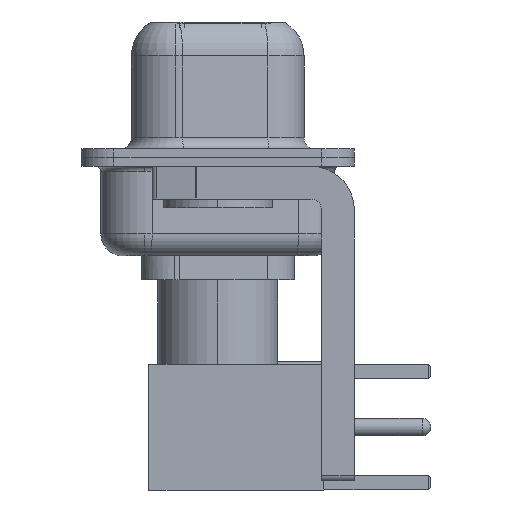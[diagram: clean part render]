
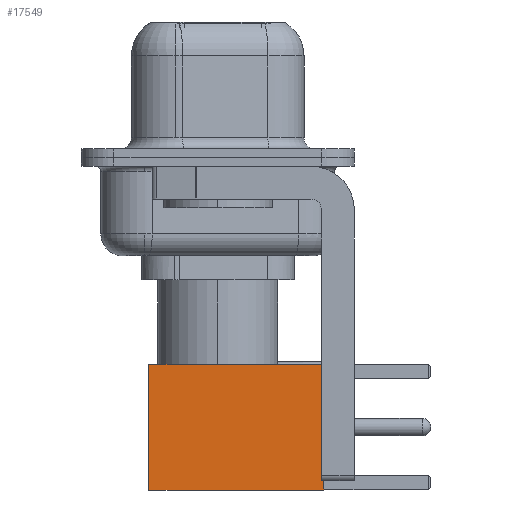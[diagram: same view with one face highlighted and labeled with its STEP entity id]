
A CAD part, left-side view. The second image highlights one B-rep face of the part: STEP entity #17549.
In plain terms, the highlighted face is planar.
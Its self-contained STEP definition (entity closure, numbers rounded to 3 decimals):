
#241 = VECTOR ( 'NONE', #1035, 1000. ) ;
#527 = CARTESIAN_POINT ( 'NONE',  ( -2.875, 2.875, 8. ) ) ;
#1035 = DIRECTION ( 'NONE',  ( 0., 0., -1. ) ) ;
#1193 = CARTESIAN_POINT ( 'NONE',  ( 2.875, 2.875, 0. ) ) ;
#1382 = DIRECTION ( 'NONE',  ( 0., 1., 0. ) ) ;
#2679 = CARTESIAN_POINT ( 'NONE',  ( 0., 2.875, 0. ) ) ;
#2826 = EDGE_CURVE ( 'NONE', #22947, #10564, #20649, .T. ) ;
#3095 = AXIS2_PLACEMENT_3D ( 'NONE', #13271, #1382, #13148 ) ;
#3259 = VERTEX_POINT ( 'NONE', #527 ) ;
#5227 = ORIENTED_EDGE ( 'NONE', *, *, #11038, .F. ) ;
#5588 = PLANE ( 'NONE',  #3095 ) ;
#5981 = DIRECTION ( 'NONE',  ( -1., 0., 0. ) ) ;
#8885 = CARTESIAN_POINT ( 'NONE',  ( 2.875, 2.875, 0. ) ) ;
#10263 = LINE ( 'NONE', #2679, #19811 ) ;
#10392 = ORIENTED_EDGE ( 'NONE', *, *, #2826, .T. ) ;
#10502 = DIRECTION ( 'NONE',  ( -1., 0., 0. ) ) ;
#10564 = VERTEX_POINT ( 'NONE', #1193 ) ;
#11038 = EDGE_CURVE ( 'NONE', #3259, #20014, #12808, .T. ) ;
#11419 = CARTESIAN_POINT ( 'NONE',  ( -2.875, 2.875, 0. ) ) ;
#11737 = LINE ( 'NONE', #15832, #12504 ) ;
#12504 = VECTOR ( 'NONE', #5981, 1000. ) ;
#12558 = VECTOR ( 'NONE', #18591, 1000. ) ;
#12704 = EDGE_CURVE ( 'NONE', #22947, #3259, #11737, .T. ) ;
#12808 = LINE ( 'NONE', #20487, #241 ) ;
#13148 = DIRECTION ( 'NONE',  ( 0., 0., 1. ) ) ;
#13271 = CARTESIAN_POINT ( 'NONE',  ( 2.875, 2.875, 0. ) ) ;
#13532 = ORIENTED_EDGE ( 'NONE', *, *, #16873, .T. ) ;
#13852 = ORIENTED_EDGE ( 'NONE', *, *, #12704, .F. ) ;
#15832 = CARTESIAN_POINT ( 'NONE',  ( 0., 2.875, 8. ) ) ;
#16873 = EDGE_CURVE ( 'NONE', #10564, #20014, #10263, .T. ) ;
#17549 = ADVANCED_FACE ( 'NONE', ( #23245 ), #5588, .T. ) ;
#18591 = DIRECTION ( 'NONE',  ( 0., 0., -1. ) ) ;
#19811 = VECTOR ( 'NONE', #10502, 1000. ) ;
#20014 = VERTEX_POINT ( 'NONE', #11419 ) ;
#20487 = CARTESIAN_POINT ( 'NONE',  ( -2.875, 2.875, 0. ) ) ;
#20649 = LINE ( 'NONE', #8885, #12558 ) ;
#20992 = EDGE_LOOP ( 'NONE', ( #10392, #13532, #5227, #13852 ) ) ;
#22947 = VERTEX_POINT ( 'NONE', #25214 ) ;
#23245 = FACE_OUTER_BOUND ( 'NONE', #20992, .T. ) ;
#25214 = CARTESIAN_POINT ( 'NONE',  ( 2.875, 2.875, 8. ) ) ;
